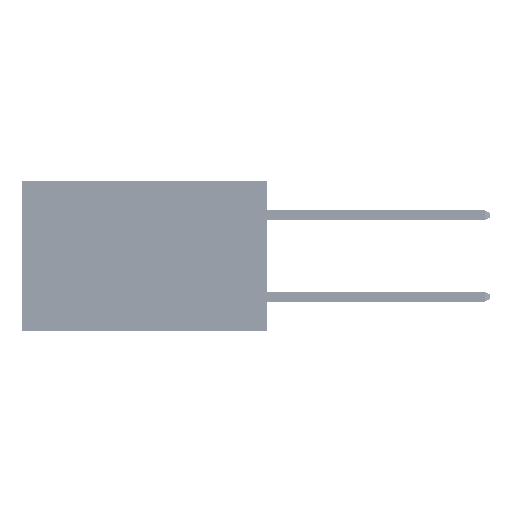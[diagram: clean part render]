
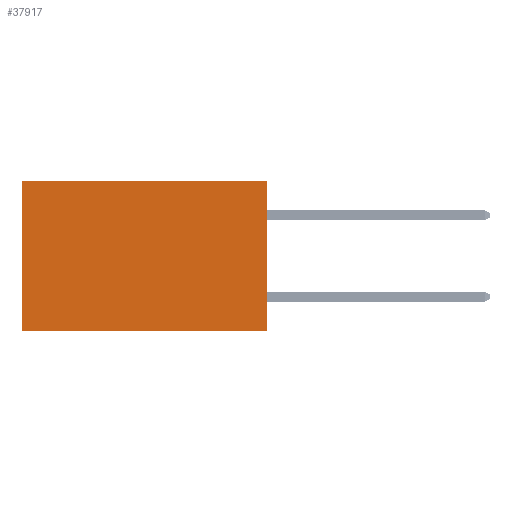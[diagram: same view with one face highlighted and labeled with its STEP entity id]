
A CAD part, left-side view. The second image highlights one B-rep face of the part: STEP entity #37917.
In plain terms, the highlighted planar face has unit normal (-1, 0, 0).
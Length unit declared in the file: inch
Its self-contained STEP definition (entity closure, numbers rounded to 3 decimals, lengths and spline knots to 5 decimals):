
#846 = AXIS2_PLACEMENT_3D ( 'NONE', #962, #23036, #26740 ) ;
#962 = CARTESIAN_POINT ( 'NONE',  ( 0.2875, 0., 0. ) ) ;
#1572 = CARTESIAN_POINT ( 'NONE',  ( 0.2875, 0.6, -0.37 ) ) ;
#1621 = DIRECTION ( 'NONE',  ( 0., 1., 0. ) ) ;
#1934 = DIRECTION ( 'NONE',  ( 0., 1., 0. ) ) ;
#2469 = VECTOR ( 'NONE', #37604, 39.37008 ) ;
#3833 = VECTOR ( 'NONE', #1934, 39.37008 ) ;
#4039 = EDGE_CURVE ( 'NONE', #17015, #30591, #43841, .T. ) ;
#8458 = VERTEX_POINT ( 'NONE', #1572 ) ;
#8831 = LINE ( 'NONE', #16783, #29000 ) ;
#12068 = ORIENTED_EDGE ( 'NONE', *, *, #32902, .F. ) ;
#14493 = VECTOR ( 'NONE', #1621, 39.37008 ) ;
#15798 = PLANE ( 'NONE',  #846 ) ;
#15945 = LINE ( 'NONE', #42303, #3833 ) ;
#16783 = CARTESIAN_POINT ( 'NONE',  ( 0.2875, 0., 0. ) ) ;
#16804 = EDGE_LOOP ( 'NONE', ( #35284, #20370, #12068, #31031 ) ) ;
#17015 = VERTEX_POINT ( 'NONE', #41768 ) ;
#20370 = ORIENTED_EDGE ( 'NONE', *, *, #38099, .F. ) ;
#23036 = DIRECTION ( 'NONE',  ( 1., 0., 0. ) ) ;
#24757 = CARTESIAN_POINT ( 'NONE',  ( 0.2875, 0., -0.37 ) ) ;
#26153 = VERTEX_POINT ( 'NONE', #24757 ) ;
#26347 = FACE_OUTER_BOUND ( 'NONE', #16804, .T. ) ;
#26740 = DIRECTION ( 'NONE',  ( 0., 0., -1. ) ) ;
#27056 = EDGE_CURVE ( 'NONE', #30591, #8458, #44493, .T. ) ;
#27548 = CARTESIAN_POINT ( 'NONE',  ( 0.2875, 0., 0. ) ) ;
#29000 = VECTOR ( 'NONE', #31552, 39.37008 ) ;
#30591 = VERTEX_POINT ( 'NONE', #40145 ) ;
#31031 = ORIENTED_EDGE ( 'NONE', *, *, #4039, .T. ) ;
#31552 = DIRECTION ( 'NONE',  ( 0., 0., -1. ) ) ;
#32902 = EDGE_CURVE ( 'NONE', #17015, #26153, #8831, .T. ) ;
#35284 = ORIENTED_EDGE ( 'NONE', *, *, #27056, .T. ) ;
#37604 = DIRECTION ( 'NONE',  ( 0., 0., -1. ) ) ;
#37917 = ADVANCED_FACE ( 'NONE', ( #26347 ), #15798, .F. ) ;
#38099 = EDGE_CURVE ( 'NONE', #26153, #8458, #15945, .T. ) ;
#40145 = CARTESIAN_POINT ( 'NONE',  ( 0.2875, 0.6, 0. ) ) ;
#41768 = CARTESIAN_POINT ( 'NONE',  ( 0.2875, 0., 0. ) ) ;
#42303 = CARTESIAN_POINT ( 'NONE',  ( 0.2875, 0., -0.37 ) ) ;
#43841 = LINE ( 'NONE', #27548, #14493 ) ;
#44493 = LINE ( 'NONE', #45205, #2469 ) ;
#45205 = CARTESIAN_POINT ( 'NONE',  ( 0.2875, 0.6, 0. ) ) ;
